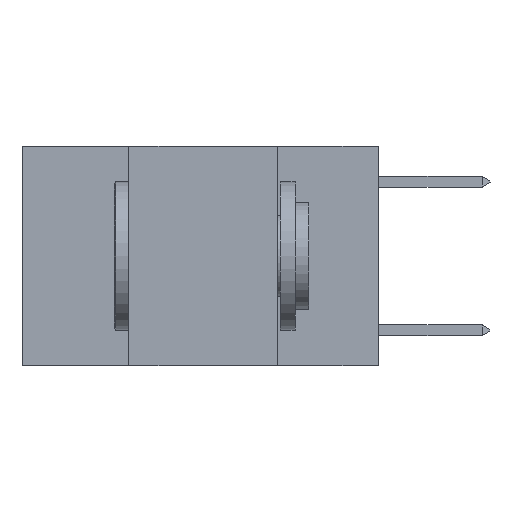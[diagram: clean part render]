
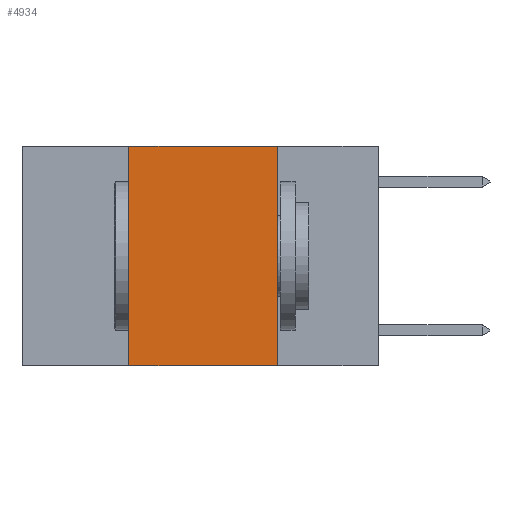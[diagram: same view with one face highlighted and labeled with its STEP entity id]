
A CAD part, left-side view. The second image highlights one B-rep face of the part: STEP entity #4934.
In plain terms, the highlighted planar face has unit normal (-1, 0, 0).
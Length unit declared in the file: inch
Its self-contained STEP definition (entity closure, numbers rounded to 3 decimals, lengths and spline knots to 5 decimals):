
#160 = LINE ( 'NONE', #6118, #8877 ) ;
#300 = EDGE_CURVE ( 'NONE', #3190, #1525, #2610, .T. ) ;
#447 = CARTESIAN_POINT ( 'NONE',  ( 0., 0.6, 0. ) ) ;
#633 = LINE ( 'NONE', #4856, #9372 ) ;
#982 = CARTESIAN_POINT ( 'NONE',  ( 0., 0.17, -0.37 ) ) ;
#1167 = AXIS2_PLACEMENT_3D ( 'NONE', #447, #11552, #11686 ) ;
#1525 = VERTEX_POINT ( 'NONE', #3162 ) ;
#2610 = LINE ( 'NONE', #6694, #7413 ) ;
#3026 = CARTESIAN_POINT ( 'NONE',  ( 0., 0.6, -0.37 ) ) ;
#3057 = EDGE_CURVE ( 'NONE', #12833, #3672, #160, .T. ) ;
#3162 = CARTESIAN_POINT ( 'NONE',  ( 0., 0.42, 0. ) ) ;
#3190 = VERTEX_POINT ( 'NONE', #8442 ) ;
#3672 = VERTEX_POINT ( 'NONE', #982 ) ;
#4381 = DIRECTION ( 'NONE',  ( 0., 0., 1. ) ) ;
#4800 = DIRECTION ( 'NONE',  ( 0., -1., 0. ) ) ;
#4856 = CARTESIAN_POINT ( 'NONE',  ( 0., 0.6, 0. ) ) ;
#4934 = ADVANCED_FACE ( 'NONE', ( #6531 ), #9637, .F. ) ;
#6118 = CARTESIAN_POINT ( 'NONE',  ( 0., 0.17, 0. ) ) ;
#6531 = FACE_OUTER_BOUND ( 'NONE', #8646, .T. ) ;
#6694 = CARTESIAN_POINT ( 'NONE',  ( 0., 0.42, 0. ) ) ;
#7064 = EDGE_CURVE ( 'NONE', #1525, #12833, #633, .T. ) ;
#7309 = CARTESIAN_POINT ( 'NONE',  ( 0., 0.17, 0. ) ) ;
#7413 = VECTOR ( 'NONE', #4381, 39.37008 ) ;
#7962 = ORIENTED_EDGE ( 'NONE', *, *, #7064, .F. ) ;
#8107 = LINE ( 'NONE', #3026, #9034 ) ;
#8442 = CARTESIAN_POINT ( 'NONE',  ( 0., 0.42, -0.37 ) ) ;
#8552 = ORIENTED_EDGE ( 'NONE', *, *, #300, .F. ) ;
#8646 = EDGE_LOOP ( 'NONE', ( #10905, #7962, #8552, #11984 ) ) ;
#8877 = VECTOR ( 'NONE', #12398, 39.37008 ) ;
#9034 = VECTOR ( 'NONE', #11203, 39.37008 ) ;
#9372 = VECTOR ( 'NONE', #4800, 39.37008 ) ;
#9637 = PLANE ( 'NONE',  #1167 ) ;
#10905 = ORIENTED_EDGE ( 'NONE', *, *, #3057, .F. ) ;
#11203 = DIRECTION ( 'NONE',  ( 0., -1., 0. ) ) ;
#11552 = DIRECTION ( 'NONE',  ( 1., 0., 0. ) ) ;
#11686 = DIRECTION ( 'NONE',  ( 0., 0., -1. ) ) ;
#11984 = ORIENTED_EDGE ( 'NONE', *, *, #13127, .T. ) ;
#12398 = DIRECTION ( 'NONE',  ( 0., 0., -1. ) ) ;
#12833 = VERTEX_POINT ( 'NONE', #7309 ) ;
#13127 = EDGE_CURVE ( 'NONE', #3190, #3672, #8107, .T. ) ;
